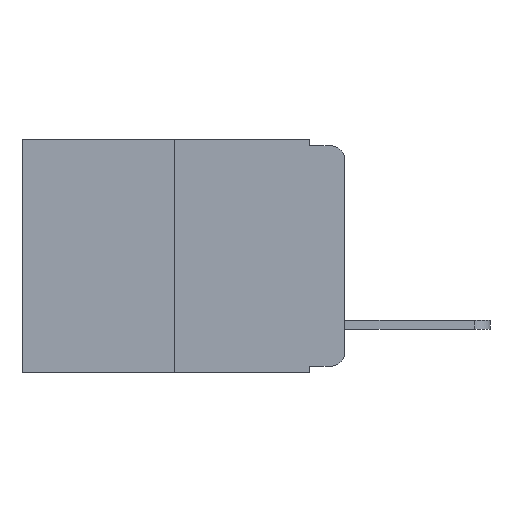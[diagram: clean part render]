
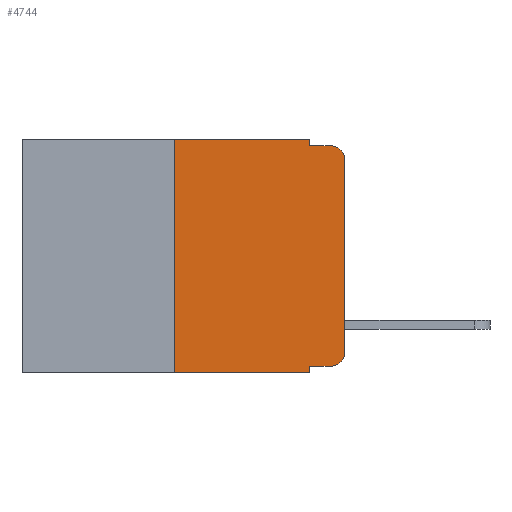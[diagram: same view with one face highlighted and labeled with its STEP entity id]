
A CAD part, left-side view. The second image highlights one B-rep face of the part: STEP entity #4744.
In plain terms, the highlighted planar face has unit normal (-1, 0, 0).
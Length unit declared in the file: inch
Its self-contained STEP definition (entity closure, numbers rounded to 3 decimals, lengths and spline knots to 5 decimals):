
#46 = AXIS2_PLACEMENT_3D ( 'NONE', #21732, #6528, #18412 ) ;
#556 = CARTESIAN_POINT ( 'NONE',  ( 0., 0.473, -0.343 ) ) ;
#582 = CARTESIAN_POINT ( 'NONE',  ( 0., 0.051, -0.333 ) ) ;
#705 = EDGE_CURVE ( 'NONE', #16573, #17741, #7444, .T. ) ;
#983 = CARTESIAN_POINT ( 'NONE',  ( 0., 0.051, -0.333 ) ) ;
#1474 = EDGE_CURVE ( 'NONE', #16197, #11681, #1811, .T. ) ;
#1811 = LINE ( 'NONE', #7012, #5832 ) ;
#2024 = VECTOR ( 'NONE', #6173, 39.37008 ) ;
#2164 = VECTOR ( 'NONE', #11109, 39.37008 ) ;
#2350 = DIRECTION ( 'NONE',  ( 0., -1., 0. ) ) ;
#2467 = ORIENTED_EDGE ( 'NONE', *, *, #19089, .F. ) ;
#2555 = AXIS2_PLACEMENT_3D ( 'NONE', #13004, #19724, #8042 ) ;
#3203 = CARTESIAN_POINT ( 'NONE',  ( 0., 0., 0. ) ) ;
#3800 = LINE ( 'NONE', #4765, #11514 ) ;
#3881 = LINE ( 'NONE', #4512, #2024 ) ;
#4444 = CARTESIAN_POINT ( 'NONE',  ( 0., 0.051, 0. ) ) ;
#4473 = ORIENTED_EDGE ( 'NONE', *, *, #9799, .T. ) ;
#4512 = CARTESIAN_POINT ( 'NONE',  ( 0., 0.051, 0. ) ) ;
#4744 = ADVANCED_FACE ( 'NONE', ( #6469 ), #6037, .F. ) ;
#4765 = CARTESIAN_POINT ( 'NONE',  ( 0., 0.473, 0. ) ) ;
#4855 = DIRECTION ( 'NONE',  ( 0., 0., 1. ) ) ;
#4936 = DIRECTION ( 'NONE',  ( -1., 0., 0. ) ) ;
#5220 = ORIENTED_EDGE ( 'NONE', *, *, #11524, .T. ) ;
#5382 = CARTESIAN_POINT ( 'NONE',  ( 0., 0.051, -0.01 ) ) ;
#5832 = VECTOR ( 'NONE', #7084, 39.37008 ) ;
#5936 = ORIENTED_EDGE ( 'NONE', *, *, #10666, .F. ) ;
#6037 = PLANE ( 'NONE',  #2555 ) ;
#6066 = DIRECTION ( 'NONE',  ( 0., 0., 1. ) ) ;
#6173 = DIRECTION ( 'NONE',  ( 0., 0., -1. ) ) ;
#6177 = EDGE_LOOP ( 'NONE', ( #16843, #15779, #2467, #17050, #12339, #7426, #19279, #5936, #4473, #5220 ) ) ;
#6469 = FACE_OUTER_BOUND ( 'NONE', #6177, .T. ) ;
#6528 = DIRECTION ( 'NONE',  ( -1., 0., 0. ) ) ;
#7012 = CARTESIAN_POINT ( 'NONE',  ( 0., 0.051, 0. ) ) ;
#7084 = DIRECTION ( 'NONE',  ( 0., 0., -1. ) ) ;
#7166 = LINE ( 'NONE', #983, #8211 ) ;
#7426 = ORIENTED_EDGE ( 'NONE', *, *, #8316, .F. ) ;
#7444 = CIRCLE ( 'NONE', #46, 0.02 ) ;
#7478 = CIRCLE ( 'NONE', #20178, 0.02 ) ;
#8018 = DIRECTION ( 'NONE',  ( 0., -1., 0. ) ) ;
#8042 = DIRECTION ( 'NONE',  ( 0., 0., -1. ) ) ;
#8211 = VECTOR ( 'NONE', #8018, 39.37008 ) ;
#8260 = VERTEX_POINT ( 'NONE', #9115 ) ;
#8316 = EDGE_CURVE ( 'NONE', #8260, #21716, #16299, .T. ) ;
#9115 = CARTESIAN_POINT ( 'NONE',  ( 0., 0.25, -0.343 ) ) ;
#9622 = EDGE_CURVE ( 'NONE', #8260, #17990, #19681, .T. ) ;
#9799 = EDGE_CURVE ( 'NONE', #11825, #11745, #7166, .T. ) ;
#10050 = DIRECTION ( 'NONE',  ( 0., 0., -1. ) ) ;
#10557 = CARTESIAN_POINT ( 'NONE',  ( 0., 0.25, 0. ) ) ;
#10666 = EDGE_CURVE ( 'NONE', #11825, #17990, #3881, .T. ) ;
#10829 = CARTESIAN_POINT ( 'NONE',  ( 0., 0., -0.03 ) ) ;
#11109 = DIRECTION ( 'NONE',  ( 0., -1., 0. ) ) ;
#11514 = VECTOR ( 'NONE', #15017, 39.37008 ) ;
#11524 = EDGE_CURVE ( 'NONE', #11745, #13207, #7478, .T. ) ;
#11681 = VERTEX_POINT ( 'NONE', #5382 ) ;
#11719 = CARTESIAN_POINT ( 'NONE',  ( 0., 0.051, -0.343 ) ) ;
#11737 = VECTOR ( 'NONE', #6066, 39.37008 ) ;
#11745 = VERTEX_POINT ( 'NONE', #12487 ) ;
#11825 = VERTEX_POINT ( 'NONE', #582 ) ;
#12339 = ORIENTED_EDGE ( 'NONE', *, *, #22038, .F. ) ;
#12487 = CARTESIAN_POINT ( 'NONE',  ( 0., 0.02, -0.333 ) ) ;
#12748 = CARTESIAN_POINT ( 'NONE',  ( 0., 0., -0.313 ) ) ;
#13004 = CARTESIAN_POINT ( 'NONE',  ( 0., 0.473, 0. ) ) ;
#13207 = VERTEX_POINT ( 'NONE', #12748 ) ;
#13689 = CARTESIAN_POINT ( 'NONE',  ( 0., 0.02, -0.01 ) ) ;
#15017 = DIRECTION ( 'NONE',  ( 0., -1., 0. ) ) ;
#15779 = ORIENTED_EDGE ( 'NONE', *, *, #705, .T. ) ;
#15803 = EDGE_CURVE ( 'NONE', #13207, #16573, #16748, .T. ) ;
#16197 = VERTEX_POINT ( 'NONE', #4444 ) ;
#16299 = LINE ( 'NONE', #19601, #11737 ) ;
#16573 = VERTEX_POINT ( 'NONE', #10829 ) ;
#16748 = LINE ( 'NONE', #3203, #20206 ) ;
#16843 = ORIENTED_EDGE ( 'NONE', *, *, #15803, .T. ) ;
#17050 = ORIENTED_EDGE ( 'NONE', *, *, #1474, .F. ) ;
#17360 = LINE ( 'NONE', #21507, #2164 ) ;
#17741 = VERTEX_POINT ( 'NONE', #13689 ) ;
#17990 = VERTEX_POINT ( 'NONE', #11719 ) ;
#18349 = VECTOR ( 'NONE', #2350, 39.37008 ) ;
#18412 = DIRECTION ( 'NONE',  ( 0., 0., -1. ) ) ;
#18547 = CARTESIAN_POINT ( 'NONE',  ( 0., 0.02, -0.313 ) ) ;
#19089 = EDGE_CURVE ( 'NONE', #11681, #17741, #17360, .T. ) ;
#19279 = ORIENTED_EDGE ( 'NONE', *, *, #9622, .T. ) ;
#19601 = CARTESIAN_POINT ( 'NONE',  ( 0., 0.25, 0. ) ) ;
#19681 = LINE ( 'NONE', #556, #18349 ) ;
#19724 = DIRECTION ( 'NONE',  ( 1., 0., 0. ) ) ;
#20178 = AXIS2_PLACEMENT_3D ( 'NONE', #18547, #4936, #10050 ) ;
#20206 = VECTOR ( 'NONE', #4855, 39.37008 ) ;
#21507 = CARTESIAN_POINT ( 'NONE',  ( 0., 0.051, -0.01 ) ) ;
#21716 = VERTEX_POINT ( 'NONE', #10557 ) ;
#21732 = CARTESIAN_POINT ( 'NONE',  ( 0., 0.02, -0.03 ) ) ;
#22038 = EDGE_CURVE ( 'NONE', #21716, #16197, #3800, .T. ) ;
